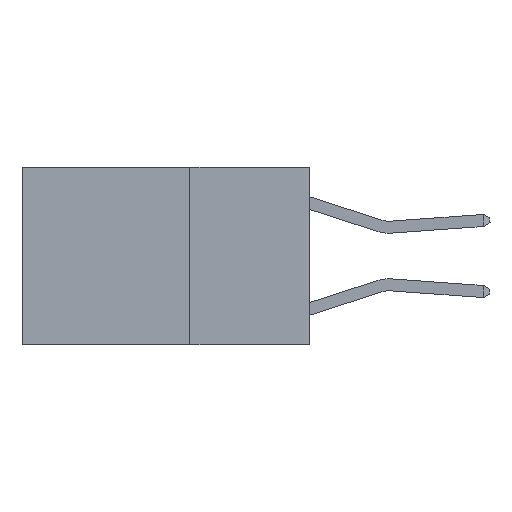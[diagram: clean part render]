
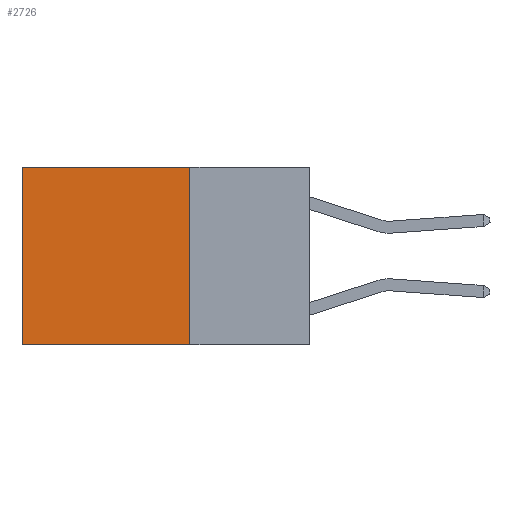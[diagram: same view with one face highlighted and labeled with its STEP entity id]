
A CAD part, left-side view. The second image highlights one B-rep face of the part: STEP entity #2726.
In plain terms, the highlighted planar face has unit normal (-1, 0, 0).
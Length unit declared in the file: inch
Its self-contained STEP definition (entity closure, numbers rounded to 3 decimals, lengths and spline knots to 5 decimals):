
#146 = VERTEX_POINT ( 'NONE', #6465 ) ;
#265 = VECTOR ( 'NONE', #5749, 39.37008 ) ;
#805 = VERTEX_POINT ( 'NONE', #6296 ) ;
#1142 = VERTEX_POINT ( 'NONE', #15302 ) ;
#2344 = ORIENTED_EDGE ( 'NONE', *, *, #6958, .T. ) ;
#2601 = CARTESIAN_POINT ( 'NONE',  ( 0.2625, 0.25, 0. ) ) ;
#2726 = ADVANCED_FACE ( 'NONE', ( #5638 ), #11696, .F. ) ;
#3630 = EDGE_LOOP ( 'NONE', ( #15440, #9061, #13503, #2344 ) ) ;
#3855 = DIRECTION ( 'NONE',  ( 0., 1., 0. ) ) ;
#5450 = LINE ( 'NONE', #11776, #11523 ) ;
#5631 = CARTESIAN_POINT ( 'NONE',  ( 0.2625, 0.6, 0. ) ) ;
#5638 = FACE_OUTER_BOUND ( 'NONE', #3630, .T. ) ;
#5749 = DIRECTION ( 'NONE',  ( 0., 0., -1. ) ) ;
#6296 = CARTESIAN_POINT ( 'NONE',  ( 0.2625, 0.25, 0. ) ) ;
#6465 = CARTESIAN_POINT ( 'NONE',  ( 0.2625, 0.6, -0.37 ) ) ;
#6814 = DIRECTION ( 'NONE',  ( 1., 0., 0. ) ) ;
#6958 = EDGE_CURVE ( 'NONE', #805, #10669, #9103, .T. ) ;
#7033 = EDGE_CURVE ( 'NONE', #805, #1142, #11236, .T. ) ;
#7535 = DIRECTION ( 'NONE',  ( 0., 0., -1. ) ) ;
#8726 = VECTOR ( 'NONE', #3855, 39.37008 ) ;
#9047 = AXIS2_PLACEMENT_3D ( 'NONE', #14184, #6814, #15371 ) ;
#9061 = ORIENTED_EDGE ( 'NONE', *, *, #12802, .F. ) ;
#9103 = LINE ( 'NONE', #2601, #8726 ) ;
#10545 = CARTESIAN_POINT ( 'NONE',  ( 0.2625, 0.6, 0. ) ) ;
#10669 = VERTEX_POINT ( 'NONE', #5631 ) ;
#10845 = VECTOR ( 'NONE', #7535, 39.37008 ) ;
#11236 = LINE ( 'NONE', #13720, #10845 ) ;
#11523 = VECTOR ( 'NONE', #13067, 39.37008 ) ;
#11696 = PLANE ( 'NONE',  #9047 ) ;
#11776 = CARTESIAN_POINT ( 'NONE',  ( 0.2625, 0.25, -0.37 ) ) ;
#12802 = EDGE_CURVE ( 'NONE', #1142, #146, #5450, .T. ) ;
#12903 = LINE ( 'NONE', #10545, #265 ) ;
#13067 = DIRECTION ( 'NONE',  ( 0., 1., 0. ) ) ;
#13346 = EDGE_CURVE ( 'NONE', #10669, #146, #12903, .T. ) ;
#13503 = ORIENTED_EDGE ( 'NONE', *, *, #7033, .F. ) ;
#13720 = CARTESIAN_POINT ( 'NONE',  ( 0.2625, 0.25, 0. ) ) ;
#14184 = CARTESIAN_POINT ( 'NONE',  ( 0.2625, 0.25, 0. ) ) ;
#15302 = CARTESIAN_POINT ( 'NONE',  ( 0.2625, 0.25, -0.37 ) ) ;
#15371 = DIRECTION ( 'NONE',  ( 0., 0., -1. ) ) ;
#15440 = ORIENTED_EDGE ( 'NONE', *, *, #13346, .T. ) ;
